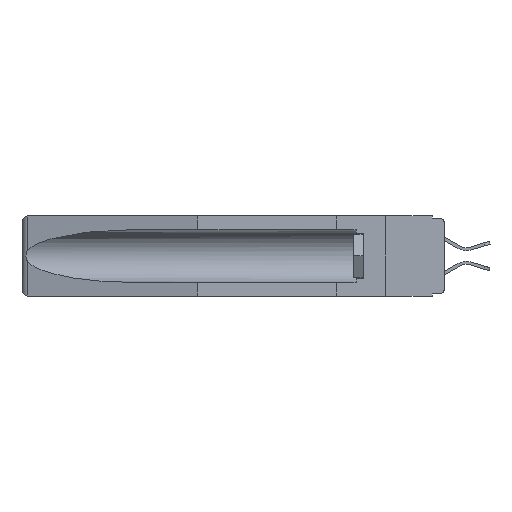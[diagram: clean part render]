
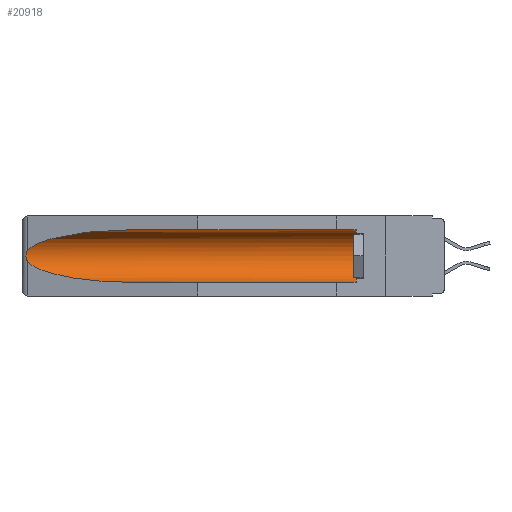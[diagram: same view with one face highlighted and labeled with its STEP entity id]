
A CAD part, left-side view. The second image highlights one B-rep face of the part: STEP entity #20918.
In plain terms, the highlighted cylindrical face has radius 2.857 mm (diameter 5.715 mm), a partial arc.
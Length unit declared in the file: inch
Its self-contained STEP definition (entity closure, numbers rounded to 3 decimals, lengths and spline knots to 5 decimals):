
#107 = ORIENTED_EDGE ( 'NONE', *, *, #24774, .F. ) ;
#838 = CARTESIAN_POINT ( 'NONE',  ( 0.26537, 1.52718, -0.14972 ) ) ;
#1128 = VERTEX_POINT ( 'NONE', #14169 ) ;
#1314 = ORIENTED_EDGE ( 'NONE', *, *, #11564, .T. ) ;
#1452 = DIRECTION ( 'NONE',  ( 0., -1., 0. ) ) ;
#2539 = CARTESIAN_POINT ( 'NONE',  ( 0.155, 1.07973, -0.059 ) ) ;
#2716 =( BOUNDED_CURVE ( )  B_SPLINE_CURVE ( 3, ( #19654, #3086, #13595, #17615 ),
 .UNSPECIFIED., .F., .F. ) 
 B_SPLINE_CURVE_WITH_KNOTS ( ( 4, 4 ),
 ( 0.1948, 1.5708 ),
 .UNSPECIFIED. ) 
 CURVE ( )  GEOMETRIC_REPRESENTATION_ITEM ( )  RATIONAL_B_SPLINE_CURVE ( ( 1., 0.848, 0.848, 1. ) ) 
 REPRESENTATION_ITEM ( '' )  );
#3010 = CARTESIAN_POINT ( 'NONE',  ( 0.155, 1.07973, -0.059 ) ) ;
#3086 = CARTESIAN_POINT ( 'NONE',  ( 0.25451, 1.48313, -0.24835 ) ) ;
#3331 = ORIENTED_EDGE ( 'NONE', *, *, #14259, .T. ) ;
#3439 = FACE_OUTER_BOUND ( 'NONE', #15557, .T. ) ;
#5186 = CARTESIAN_POINT ( 'NONE',  ( 0.26655, 1.53094, -0.18657 ) ) ;
#5309 = CARTESIAN_POINT ( 'NONE',  ( 0.155, -0.30754, -0.059 ) ) ;
#7369 = CARTESIAN_POINT ( 'NONE',  ( 0.26537, 1.52718, -0.14972 ) ) ;
#7538 = B_SPLINE_CURVE_WITH_KNOTS ( 'NONE', 3,
 ( #838, #19589, #9192, #23730, #11273, #25812, #17633, #5186, #23917, #11449 ),
 .UNSPECIFIED., .F., .F.,
 ( 4, 2, 2, 2, 4 ),
 ( 0., 0.00029, 0.00058, 0.00087, 0.00117 ),
 .UNSPECIFIED. ) ;
#7715 = CARTESIAN_POINT ( 'NONE',  ( 0.155, -0.30754, -0.284 ) ) ;
#7886 = DIRECTION ( 'NONE',  ( 0., 1., 0. ) ) ;
#8081 = CIRCLE ( 'NONE', #11089, 0.1125 ) ;
#8094 = EDGE_CURVE ( 'NONE', #20685, #1128, #8081, .T. ) ;
#8115 = LINE ( 'NONE', #7715, #10080 ) ;
#8369 = CARTESIAN_POINT ( 'NONE',  ( 0.155, -0.30754, -0.1715 ) ) ;
#8430 = DIRECTION ( 'NONE',  ( 0., 0., 1. ) ) ;
#8485 = VERTEX_POINT ( 'NONE', #15676 ) ;
#8896 = EDGE_CURVE ( 'NONE', #1128, #19809, #9659, .T. ) ;
#9192 = CARTESIAN_POINT ( 'NONE',  ( 0.26654, 1.53092, -0.15636 ) ) ;
#9240 = ORIENTED_EDGE ( 'NONE', *, *, #13733, .T. ) ;
#9562 = CARTESIAN_POINT ( 'NONE',  ( 0.21114, 1.30732, -0.059 ) ) ;
#9659 = LINE ( 'NONE', #5309, #21034 ) ;
#9780 = AXIS2_PLACEMENT_3D ( 'NONE', #8369, #22901, #10455 ) ;
#10080 = VECTOR ( 'NONE', #7886, 39.37008 ) ;
#10455 = DIRECTION ( 'NONE',  ( 0., 0., 1. ) ) ;
#11089 = AXIS2_PLACEMENT_3D ( 'NONE', #11786, #1452, #8430 ) ;
#11273 = CARTESIAN_POINT ( 'NONE',  ( 0.2675, 1.53308, -0.16763 ) ) ;
#11449 = CARTESIAN_POINT ( 'NONE',  ( 0.26537, 1.52718, -0.19328 ) ) ;
#11564 = EDGE_CURVE ( 'NONE', #19809, #25504, #13856, .T. ) ;
#11786 = CARTESIAN_POINT ( 'NONE',  ( 0.155, 0.126, -0.1715 ) ) ;
#12437 = ORIENTED_EDGE ( 'NONE', *, *, #8896, .T. ) ;
#13239 = CARTESIAN_POINT ( 'NONE',  ( 0.155, 1.07973, -0.284 ) ) ;
#13595 = CARTESIAN_POINT ( 'NONE',  ( 0.21114, 1.30732, -0.284 ) ) ;
#13733 = EDGE_CURVE ( 'NONE', #25504, #8485, #7538, .T. ) ;
#13856 =( BOUNDED_CURVE ( )  B_SPLINE_CURVE ( 3, ( #3010, #9562, #24082, #7369 ),
 .UNSPECIFIED., .F., .F. ) 
 B_SPLINE_CURVE_WITH_KNOTS ( ( 4, 4 ),
 ( 4.71239, 6.08839 ),
 .UNSPECIFIED. ) 
 CURVE ( )  GEOMETRIC_REPRESENTATION_ITEM ( )  RATIONAL_B_SPLINE_CURVE ( ( 1., 0.848, 0.848, 1. ) ) 
 REPRESENTATION_ITEM ( '' )  );
#14169 = CARTESIAN_POINT ( 'NONE',  ( 0.155, 0.126, -0.059 ) ) ;
#14259 = EDGE_CURVE ( 'NONE', #8485, #21104, #2716, .T. ) ;
#15557 = EDGE_LOOP ( 'NONE', ( #1314, #9240, #3331, #107, #24931, #12437 ) ) ;
#15676 = CARTESIAN_POINT ( 'NONE',  ( 0.26537, 1.52718, -0.19328 ) ) ;
#15917 = CARTESIAN_POINT ( 'NONE',  ( 0.155, 0.126, -0.284 ) ) ;
#17615 = CARTESIAN_POINT ( 'NONE',  ( 0.155, 1.07973, -0.284 ) ) ;
#17633 = CARTESIAN_POINT ( 'NONE',  ( 0.2673, 1.53269, -0.17917 ) ) ;
#19589 = CARTESIAN_POINT ( 'NONE',  ( 0.26597, 1.52961, -0.15275 ) ) ;
#19654 = CARTESIAN_POINT ( 'NONE',  ( 0.26537, 1.52718, -0.19328 ) ) ;
#19809 = VERTEX_POINT ( 'NONE', #2539 ) ;
#20063 = CYLINDRICAL_SURFACE ( 'NONE', #9780, 0.1125 ) ;
#20685 = VERTEX_POINT ( 'NONE', #15917 ) ;
#20918 = ADVANCED_FACE ( 'NONE', ( #3439 ), #20063, .F. ) ;
#21034 = VECTOR ( 'NONE', #21585, 39.37008 ) ;
#21104 = VERTEX_POINT ( 'NONE', #13239 ) ;
#21585 = DIRECTION ( 'NONE',  ( 0., 1., 0. ) ) ;
#22310 = CARTESIAN_POINT ( 'NONE',  ( 0.26537, 1.52718, -0.14972 ) ) ;
#22901 = DIRECTION ( 'NONE',  ( 0., 1., 0. ) ) ;
#23730 = CARTESIAN_POINT ( 'NONE',  ( 0.2673, 1.5327, -0.16383 ) ) ;
#23917 = CARTESIAN_POINT ( 'NONE',  ( 0.26597, 1.5296, -0.19026 ) ) ;
#24082 = CARTESIAN_POINT ( 'NONE',  ( 0.25451, 1.48313, -0.09465 ) ) ;
#24774 = EDGE_CURVE ( 'NONE', #20685, #21104, #8115, .T. ) ;
#24931 = ORIENTED_EDGE ( 'NONE', *, *, #8094, .T. ) ;
#25504 = VERTEX_POINT ( 'NONE', #22310 ) ;
#25812 = CARTESIAN_POINT ( 'NONE',  ( 0.2675, 1.53308, -0.17534 ) ) ;
